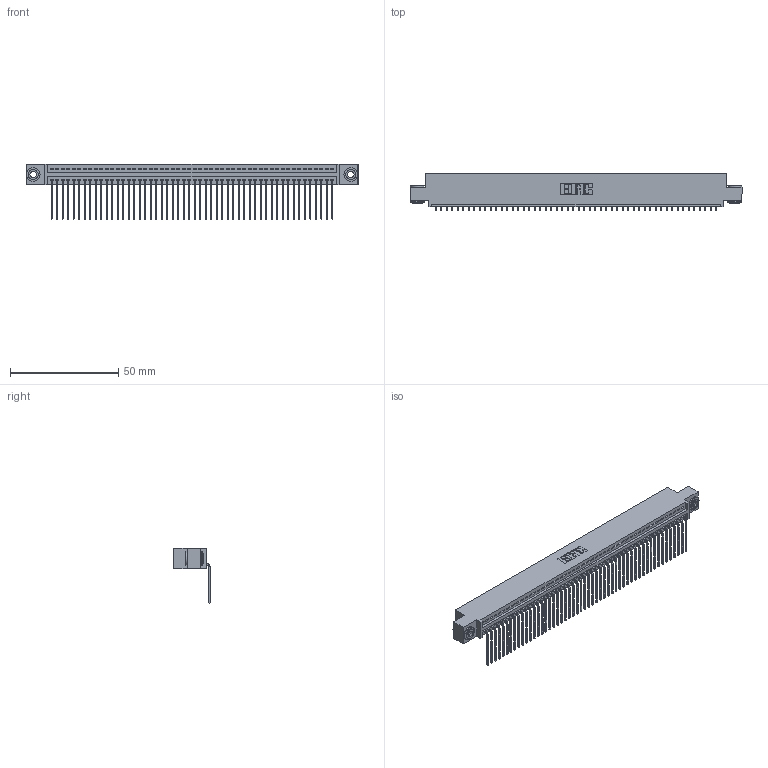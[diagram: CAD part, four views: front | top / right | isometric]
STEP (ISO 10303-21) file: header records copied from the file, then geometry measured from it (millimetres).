
FILE_DESCRIPTION (( 'STEP AP203' ), '1' );
FILE_NAME ('395-052-559-403.STEP', '2018-11-21T02:06:12', ( '' ), ( '' ), 'SwSTEP 2.0', 'SolidWorks 2016', '' );
FILE_SCHEMA (( 'CONFIG_CONTROL_DESIGN' ));
Length unit declared in the file: inch
Products named in the file (4): 395-052-559-403; 345-250-002_345-250-002-102; 345 Part_0.110 Offset - 0.156 Dia-TH; 345-292-001_558 559 Tail - 1
Assembly tree (55 placements, depth 2):
  395-052-559-403
    345 Part_0.110 Offset - 0.156 Dia-TH
    345-292-001_558 559 Tail - 1  x52
    345-250-002_345-250-002-102  x2
Bounding box: 153.29 x 16.75 x 25.53 mm (x, y, z)
Volume: 14760.7 mm3; surface area: 21066 mm2
Topology: 55 solids, 55 shells, 3288 faces, 9893 edges, 6522 vertices
Faces by surface type: plane 2278, cylinder 1002, cone 8
Entity records: 38656 total; most frequent: CARTESIAN_POINT 6675, ORIENTED_EDGE 6654, DIRECTION 5845, EDGE_CURVE 3327, LINE 2963, VECTOR 2963, VERTEX_POINT 2214, AXIS2_PLACEMENT_3D 1441
